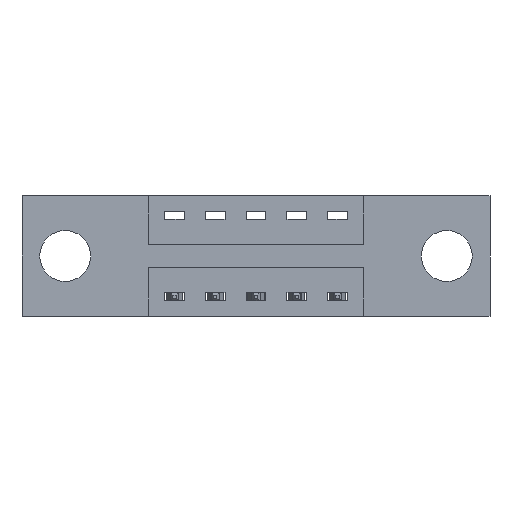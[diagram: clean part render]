
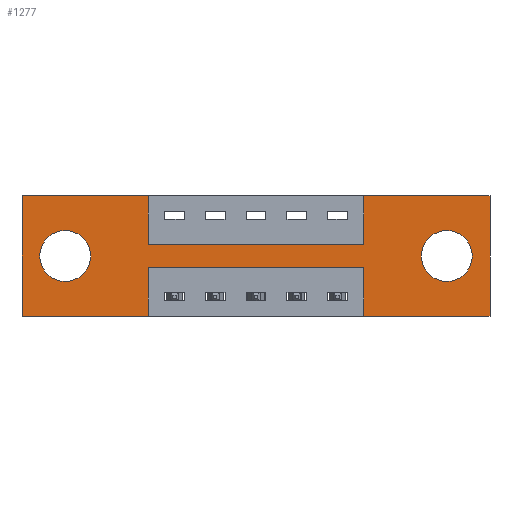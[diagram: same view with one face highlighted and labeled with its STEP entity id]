
A CAD part, front view. The second image highlights one B-rep face of the part: STEP entity #1277.
In plain terms, the highlighted planar face has unit normal (0, -1, 0).
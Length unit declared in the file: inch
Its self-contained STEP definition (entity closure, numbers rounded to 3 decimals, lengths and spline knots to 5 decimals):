
#11 = VERTEX_POINT ( 'NONE', #5093 ) ;
#17 = CARTESIAN_POINT ( 'NONE',  ( 0., 0., 0. ) ) ;
#81 = CARTESIAN_POINT ( 'NONE',  ( 1.0475, 0., -0.37 ) ) ;
#150 = CARTESIAN_POINT ( 'NONE',  ( 0.3875, 0., 0. ) ) ;
#256 = VERTEX_POINT ( 'NONE', #2211 ) ;
#365 = ORIENTED_EDGE ( 'NONE', *, *, #2794, .T. ) ;
#369 = ORIENTED_EDGE ( 'NONE', *, *, #2486, .F. ) ;
#391 = EDGE_CURVE ( 'NONE', #4098, #8076, #576, .T. ) ;
#413 = CARTESIAN_POINT ( 'NONE',  ( 0.3875, 0., 0. ) ) ;
#515 = DIRECTION ( 'NONE',  ( 0., 0., 1. ) ) ;
#557 = VERTEX_POINT ( 'NONE', #81 ) ;
#576 = LINE ( 'NONE', #939, #821 ) ;
#599 = DIRECTION ( 'NONE',  ( 0., 0., 1. ) ) ;
#690 = CARTESIAN_POINT ( 'NONE',  ( 1.0475, 0., -0.37 ) ) ;
#693 = DIRECTION ( 'NONE',  ( 0., 0., -1. ) ) ;
#708 = VERTEX_POINT ( 'NONE', #4129 ) ;
#807 = CARTESIAN_POINT ( 'NONE',  ( 0.3875, 0., -0.37 ) ) ;
#821 = VECTOR ( 'NONE', #4065, 39.37008 ) ;
#826 = VERTEX_POINT ( 'NONE', #6195 ) ;
#873 = DIRECTION ( 'NONE',  ( -1., 0., 0. ) ) ;
#936 = CARTESIAN_POINT ( 'NONE',  ( 0.3875, 0., -0.22 ) ) ;
#939 = CARTESIAN_POINT ( 'NONE',  ( 1.0475, 0., 0. ) ) ;
#938 = CARTESIAN_POINT ( 'NONE',  ( 0., 0., -0.37 ) ) ;
#969 = ORIENTED_EDGE ( 'NONE', *, *, #1299, .F. ) ;
#1014 = CIRCLE ( 'NONE', #3443, 0.078 ) ;
#1093 = VERTEX_POINT ( 'NONE', #2683 ) ;
#1226 = DIRECTION ( 'NONE',  ( 0., 0., -1. ) ) ;
#1254 = CIRCLE ( 'NONE', #3454, 0.078 ) ;
#1277 = ADVANCED_FACE ( 'NONE', ( #5258, #5063, #5084 ), #2262, .T. ) ;
#1285 = ORIENTED_EDGE ( 'NONE', *, *, #6958, .F. ) ;
#1299 = EDGE_CURVE ( 'NONE', #2511, #5468, #4144, .T. ) ;
#1366 = ORIENTED_EDGE ( 'NONE', *, *, #2957, .F. ) ;
#1419 = EDGE_CURVE ( 'NONE', #11, #5568, #1950, .T. ) ;
#1596 = DIRECTION ( 'NONE',  ( 0., 0., 1. ) ) ;
#1605 = DIRECTION ( 'NONE',  ( 0., 1., 0. ) ) ;
#1622 = CARTESIAN_POINT ( 'NONE',  ( 0.1325, 0., -0.185 ) ) ;
#1628 = ORIENTED_EDGE ( 'NONE', *, *, #5738, .F. ) ;
#1629 = ORIENTED_EDGE ( 'NONE', *, *, #6325, .T. ) ;
#1668 = VERTEX_POINT ( 'NONE', #6385 ) ;
#1729 = DIRECTION ( 'NONE',  ( 0., 0., 1. ) ) ;
#1747 = ORIENTED_EDGE ( 'NONE', *, *, #2202, .T. ) ;
#1766 = DIRECTION ( 'NONE',  ( 0., 1., 0. ) ) ;
#1792 = ORIENTED_EDGE ( 'NONE', *, *, #6989, .F. ) ;
#1818 = VERTEX_POINT ( 'NONE', #4296 ) ;
#1843 = CARTESIAN_POINT ( 'NONE',  ( 0.1325, 0., -0.185 ) ) ;
#1928 = VECTOR ( 'NONE', #7446, 39.37008 ) ;
#1950 = LINE ( 'NONE', #7511, #1928 ) ;
#1966 = DIRECTION ( 'NONE',  ( 0., 0., -1. ) ) ;
#2042 = DIRECTION ( 'NONE',  ( 0., -1., 0. ) ) ;
#2093 = CARTESIAN_POINT ( 'NONE',  ( 1.435, 0., 0. ) ) ;
#2101 = CARTESIAN_POINT ( 'NONE',  ( 0., 0., -0.37 ) ) ;
#2168 = CARTESIAN_POINT ( 'NONE',  ( 0., 0., -0.37 ) ) ;
#2202 = EDGE_CURVE ( 'NONE', #3794, #826, #7550, .T. ) ;
#2211 = CARTESIAN_POINT ( 'NONE',  ( 1.3025, 0., -0.107 ) ) ;
#2262 = PLANE ( 'NONE',  #4179 ) ;
#2295 = EDGE_LOOP ( 'NONE', ( #365, #1629 ) ) ;
#2325 = EDGE_CURVE ( 'NONE', #557, #11, #2444, .T. ) ;
#2344 = DIRECTION ( 'NONE',  ( 1., 0., 0. ) ) ;
#2400 = CARTESIAN_POINT ( 'NONE',  ( 0.1325, 0., -0.107 ) ) ;
#2416 = VECTOR ( 'NONE', #8122, 39.37008 ) ;
#2427 = DIRECTION ( 'NONE',  ( 0., 0., -1. ) ) ;
#2444 = LINE ( 'NONE', #690, #3235 ) ;
#2455 = DIRECTION ( 'NONE',  ( 0., 1., 0. ) ) ;
#2464 = CARTESIAN_POINT ( 'NONE',  ( 1.3025, 0., -0.185 ) ) ;
#2486 = EDGE_CURVE ( 'NONE', #708, #1818, #7718, .T. ) ;
#2511 = VERTEX_POINT ( 'NONE', #6304 ) ;
#2609 = EDGE_CURVE ( 'NONE', #1093, #4098, #6285, .T. ) ;
#2631 = LINE ( 'NONE', #4650, #2416 ) ;
#2683 = CARTESIAN_POINT ( 'NONE',  ( 0.3875, 0., -0.15 ) ) ;
#2726 = CIRCLE ( 'NONE', #4010, 0.078 ) ;
#2751 = ORIENTED_EDGE ( 'NONE', *, *, #391, .F. ) ;
#2794 = EDGE_CURVE ( 'NONE', #256, #7569, #2726, .T. ) ;
#2957 = EDGE_CURVE ( 'NONE', #5468, #1668, #8056, .T. ) ;
#2959 = ORIENTED_EDGE ( 'NONE', *, *, #2609, .F. ) ;
#2979 = VECTOR ( 'NONE', #7053, 39.37008 ) ;
#2994 = CARTESIAN_POINT ( 'NONE',  ( 0.3875, 0., -0.15 ) ) ;
#3079 = LINE ( 'NONE', #3340, #2979 ) ;
#3235 = VECTOR ( 'NONE', #599, 39.37008 ) ;
#3340 = CARTESIAN_POINT ( 'NONE',  ( 0., 0., 0. ) ) ;
#3443 = AXIS2_PLACEMENT_3D ( 'NONE', #1622, #1605, #1596 ) ;
#3454 = AXIS2_PLACEMENT_3D ( 'NONE', #2464, #2455, #2427 ) ;
#3777 = CARTESIAN_POINT ( 'NONE',  ( 1.3025, 0., -0.263 ) ) ;
#3794 = VERTEX_POINT ( 'NONE', #2400 ) ;
#3809 = ORIENTED_EDGE ( 'NONE', *, *, #5069, .F. ) ;
#4010 = AXIS2_PLACEMENT_3D ( 'NONE', #5011, #5445, #5435 ) ;
#4054 = AXIS2_PLACEMENT_3D ( 'NONE', #1843, #1766, #1729 ) ;
#4065 = DIRECTION ( 'NONE',  ( 0., 0., 1. ) ) ;
#4098 = VERTEX_POINT ( 'NONE', #6792 ) ;
#4129 = CARTESIAN_POINT ( 'NONE',  ( 1.435, 0., 0. ) ) ;
#4144 = LINE ( 'NONE', #938, #4336 ) ;
#4179 = AXIS2_PLACEMENT_3D ( 'NONE', #2101, #2042, #1966 ) ;
#4247 = ORIENTED_EDGE ( 'NONE', *, *, #1419, .F. ) ;
#4296 = CARTESIAN_POINT ( 'NONE',  ( 1.435, 0., -0.37 ) ) ;
#4336 = VECTOR ( 'NONE', #873, 39.37008 ) ;
#4339 = ORIENTED_EDGE ( 'NONE', *, *, #6392, .T. ) ;
#4474 = ORIENTED_EDGE ( 'NONE', *, *, #2325, .F. ) ;
#4490 = VERTEX_POINT ( 'NONE', #150 ) ;
#4650 = CARTESIAN_POINT ( 'NONE',  ( 0., 0., 0. ) ) ;
#5011 = CARTESIAN_POINT ( 'NONE',  ( 1.3025, 0., -0.185 ) ) ;
#5063 = FACE_BOUND ( 'NONE', #8064, .T. ) ;
#5069 = EDGE_CURVE ( 'NONE', #1818, #557, #6843, .T. ) ;
#5084 = FACE_OUTER_BOUND ( 'NONE', #6003, .T. ) ;
#5093 = CARTESIAN_POINT ( 'NONE',  ( 1.0475, 0., -0.22 ) ) ;
#5190 = VECTOR ( 'NONE', #7868, 39.37008 ) ;
#5238 = LINE ( 'NONE', #413, #5190 ) ;
#5258 = FACE_BOUND ( 'NONE', #2295, .T. ) ;
#5322 = VECTOR ( 'NONE', #693, 39.37008 ) ;
#5435 = DIRECTION ( 'NONE',  ( 0., 0., -1. ) ) ;
#5441 = LINE ( 'NONE', #807, #5322 ) ;
#5445 = DIRECTION ( 'NONE',  ( 0., 1., 0. ) ) ;
#5468 = VERTEX_POINT ( 'NONE', #2168 ) ;
#5535 = VECTOR ( 'NONE', #2344, 39.37008 ) ;
#5568 = VERTEX_POINT ( 'NONE', #936 ) ;
#5623 = EDGE_CURVE ( 'NONE', #5568, #2511, #5441, .T. ) ;
#5701 = ORIENTED_EDGE ( 'NONE', *, *, #5623, .F. ) ;
#5738 = EDGE_CURVE ( 'NONE', #4490, #1093, #5238, .T. ) ;
#6003 = EDGE_LOOP ( 'NONE', ( #5701, #4247, #4474, #3809, #369, #1792, #2751, #2959, #1628, #1285, #1366, #969 ) ) ;
#6110 = CARTESIAN_POINT ( 'NONE',  ( 1.0475, 0., 0. ) ) ;
#6180 = DIRECTION ( 'NONE',  ( -1., 0., 0. ) ) ;
#6194 = CARTESIAN_POINT ( 'NONE',  ( 0., 0., -0.37 ) ) ;
#6195 = CARTESIAN_POINT ( 'NONE',  ( 0.1325, 0., -0.263 ) ) ;
#6198 = VECTOR ( 'NONE', #6180, 39.37008 ) ;
#6285 = LINE ( 'NONE', #2994, #5535 ) ;
#6304 = CARTESIAN_POINT ( 'NONE',  ( 0.3875, 0., -0.37 ) ) ;
#6325 = EDGE_CURVE ( 'NONE', #7569, #256, #1254, .T. ) ;
#6385 = CARTESIAN_POINT ( 'NONE',  ( 0., 0., 0. ) ) ;
#6392 = EDGE_CURVE ( 'NONE', #826, #3794, #1014, .T. ) ;
#6792 = CARTESIAN_POINT ( 'NONE',  ( 1.0475, 0., -0.15 ) ) ;
#6843 = LINE ( 'NONE', #6194, #6198 ) ;
#6958 = EDGE_CURVE ( 'NONE', #1668, #4490, #3079, .T. ) ;
#6989 = EDGE_CURVE ( 'NONE', #8076, #708, #2631, .T. ) ;
#7053 = DIRECTION ( 'NONE',  ( 1., 0., 0. ) ) ;
#7076 = VECTOR ( 'NONE', #1226, 39.37008 ) ;
#7341 = VECTOR ( 'NONE', #515, 39.37008 ) ;
#7446 = DIRECTION ( 'NONE',  ( -1., 0., 0. ) ) ;
#7511 = CARTESIAN_POINT ( 'NONE',  ( 0.3875, 0., -0.22 ) ) ;
#7550 = CIRCLE ( 'NONE', #4054, 0.078 ) ;
#7569 = VERTEX_POINT ( 'NONE', #3777 ) ;
#7718 = LINE ( 'NONE', #2093, #7076 ) ;
#7868 = DIRECTION ( 'NONE',  ( 0., 0., -1. ) ) ;
#8056 = LINE ( 'NONE', #17, #7341 ) ;
#8064 = EDGE_LOOP ( 'NONE', ( #1747, #4339 ) ) ;
#8076 = VERTEX_POINT ( 'NONE', #6110 ) ;
#8122 = DIRECTION ( 'NONE',  ( 1., 0., 0. ) ) ;
